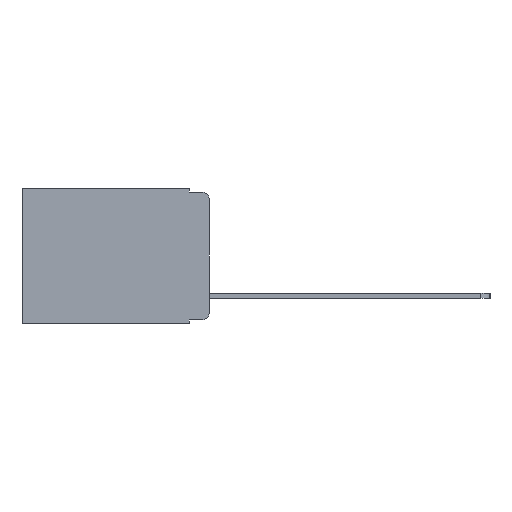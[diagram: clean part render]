
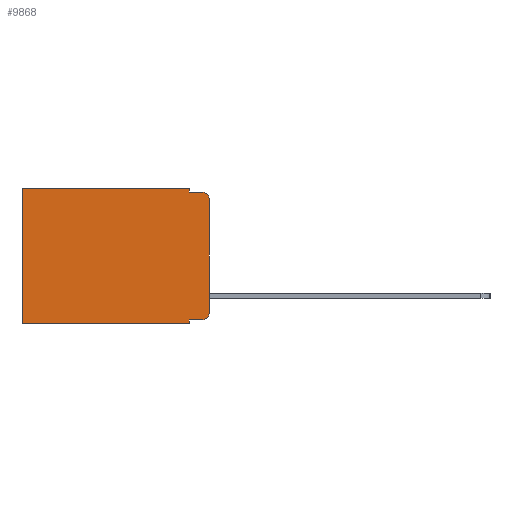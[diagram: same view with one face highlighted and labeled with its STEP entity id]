
A CAD part, left-side view. The second image highlights one B-rep face of the part: STEP entity #9868.
In plain terms, the highlighted planar face has unit normal (-1, 0, 0).
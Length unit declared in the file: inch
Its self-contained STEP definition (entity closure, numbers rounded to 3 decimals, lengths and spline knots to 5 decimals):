
#211 = CIRCLE ( 'NONE', #6795, 0.02 ) ;
#214 = DIRECTION ( 'NONE',  ( 0., 0., -1. ) ) ;
#392 = EDGE_LOOP ( 'NONE', ( #5761, #15468, #3379, #691, #3749, #3781, #10370, #563, #17552, #18116 ) ) ;
#563 = ORIENTED_EDGE ( 'NONE', *, *, #8234, .F. ) ;
#691 = ORIENTED_EDGE ( 'NONE', *, *, #2134, .F. ) ;
#769 = VERTEX_POINT ( 'NONE', #20588 ) ;
#883 = LINE ( 'NONE', #5434, #8383 ) ;
#1494 = CARTESIAN_POINT ( 'NONE',  ( 0.298, 0.051, -0.333 ) ) ;
#1606 = VERTEX_POINT ( 'NONE', #17451 ) ;
#1775 = CARTESIAN_POINT ( 'NONE',  ( 0.298, 0., -0.313 ) ) ;
#2134 = EDGE_CURVE ( 'NONE', #8348, #769, #4140, .T. ) ;
#2448 = LINE ( 'NONE', #13159, #6383 ) ;
#2516 = EDGE_CURVE ( 'NONE', #15425, #16596, #6400, .T. ) ;
#2732 = VECTOR ( 'NONE', #13446, 39.37008 ) ;
#3138 = CARTESIAN_POINT ( 'NONE',  ( 0.298, 0.051, 0. ) ) ;
#3336 = EDGE_CURVE ( 'NONE', #769, #10612, #2448, .T. ) ;
#3379 = ORIENTED_EDGE ( 'NONE', *, *, #3336, .F. ) ;
#3578 = CARTESIAN_POINT ( 'NONE',  ( 0.298, 0.051, -0.333 ) ) ;
#3749 = ORIENTED_EDGE ( 'NONE', *, *, #12738, .T. ) ;
#3781 = ORIENTED_EDGE ( 'NONE', *, *, #2516, .T. ) ;
#4140 = LINE ( 'NONE', #3138, #11976 ) ;
#4147 = CIRCLE ( 'NONE', #16805, 0.02 ) ;
#4214 = VERTEX_POINT ( 'NONE', #6397 ) ;
#4474 = VECTOR ( 'NONE', #13524, 39.37008 ) ;
#5371 = LINE ( 'NONE', #6850, #9315 ) ;
#5434 = CARTESIAN_POINT ( 'NONE',  ( 0.298, 0.051, 0. ) ) ;
#5755 = DIRECTION ( 'NONE',  ( 0., -1., 0. ) ) ;
#5761 = ORIENTED_EDGE ( 'NONE', *, *, #11861, .F. ) ;
#6383 = VECTOR ( 'NONE', #5755, 39.37008 ) ;
#6397 = CARTESIAN_POINT ( 'NONE',  ( 0.298, 0., -0.03 ) ) ;
#6400 = LINE ( 'NONE', #15675, #14639 ) ;
#6649 = FACE_OUTER_BOUND ( 'NONE', #392, .T. ) ;
#6795 = AXIS2_PLACEMENT_3D ( 'NONE', #17833, #8490, #19300 ) ;
#6850 = CARTESIAN_POINT ( 'NONE',  ( 0.298, 0., 0. ) ) ;
#6975 = DIRECTION ( 'NONE',  ( -1., 0., 0. ) ) ;
#7296 = CARTESIAN_POINT ( 'NONE',  ( 0.298, 0., 0. ) ) ;
#7990 = VERTEX_POINT ( 'NONE', #1494 ) ;
#8234 = EDGE_CURVE ( 'NONE', #7990, #1606, #883, .T. ) ;
#8348 = VERTEX_POINT ( 'NONE', #16875 ) ;
#8383 = VECTOR ( 'NONE', #214, 39.37008 ) ;
#8490 = DIRECTION ( 'NONE',  ( -1., 0., 0. ) ) ;
#8997 = DIRECTION ( 'NONE',  ( 1., 0., 0. ) ) ;
#9207 = CARTESIAN_POINT ( 'NONE',  ( 0.298, 0.02, -0.333 ) ) ;
#9315 = VECTOR ( 'NONE', #14993, 39.37008 ) ;
#9367 = VERTEX_POINT ( 'NONE', #9207 ) ;
#9449 = LINE ( 'NONE', #3578, #4474 ) ;
#9749 = EDGE_CURVE ( 'NONE', #9367, #16050, #211, .T. ) ;
#9868 = ADVANCED_FACE ( 'NONE', ( #6649 ), #16813, .F. ) ;
#10251 = VECTOR ( 'NONE', #19483, 39.37008 ) ;
#10370 = ORIENTED_EDGE ( 'NONE', *, *, #15253, .F. ) ;
#10612 = VERTEX_POINT ( 'NONE', #20762 ) ;
#11183 = CARTESIAN_POINT ( 'NONE',  ( 0.298, 0.473, -0.343 ) ) ;
#11581 = DIRECTION ( 'NONE',  ( 0., 0., -1. ) ) ;
#11861 = EDGE_CURVE ( 'NONE', #4214, #16050, #19175, .T. ) ;
#11976 = VECTOR ( 'NONE', #11581, 39.37008 ) ;
#12738 = EDGE_CURVE ( 'NONE', #8348, #15425, #5371, .T. ) ;
#13159 = CARTESIAN_POINT ( 'NONE',  ( 0.298, 0.051, -0.01 ) ) ;
#13446 = DIRECTION ( 'NONE',  ( 0., 0., -1. ) ) ;
#13524 = DIRECTION ( 'NONE',  ( 0., -1., 0. ) ) ;
#13968 = CARTESIAN_POINT ( 'NONE',  ( 0.298, 0.473, 0. ) ) ;
#14639 = VECTOR ( 'NONE', #17300, 39.37008 ) ;
#14993 = DIRECTION ( 'NONE',  ( 0., 1., 0. ) ) ;
#15253 = EDGE_CURVE ( 'NONE', #1606, #16596, #17922, .T. ) ;
#15425 = VERTEX_POINT ( 'NONE', #13968 ) ;
#15468 = ORIENTED_EDGE ( 'NONE', *, *, #19148, .T. ) ;
#15675 = CARTESIAN_POINT ( 'NONE',  ( 0.298, 0.473, 0. ) ) ;
#16044 = EDGE_CURVE ( 'NONE', #7990, #9367, #9449, .T. ) ;
#16050 = VERTEX_POINT ( 'NONE', #1775 ) ;
#16113 = AXIS2_PLACEMENT_3D ( 'NONE', #7296, #8997, #19743 ) ;
#16401 = CARTESIAN_POINT ( 'NONE',  ( 0.298, 0., 0. ) ) ;
#16551 = CARTESIAN_POINT ( 'NONE',  ( 0.298, 0.02, -0.03 ) ) ;
#16596 = VERTEX_POINT ( 'NONE', #11183 ) ;
#16805 = AXIS2_PLACEMENT_3D ( 'NONE', #16551, #6975, #18020 ) ;
#16813 = PLANE ( 'NONE',  #16113 ) ;
#16875 = CARTESIAN_POINT ( 'NONE',  ( 0.298, 0.051, 0. ) ) ;
#17300 = DIRECTION ( 'NONE',  ( 0., 0., -1. ) ) ;
#17451 = CARTESIAN_POINT ( 'NONE',  ( 0.298, 0.051, -0.343 ) ) ;
#17552 = ORIENTED_EDGE ( 'NONE', *, *, #16044, .T. ) ;
#17833 = CARTESIAN_POINT ( 'NONE',  ( 0.298, 0.02, -0.313 ) ) ;
#17922 = LINE ( 'NONE', #18028, #10251 ) ;
#18020 = DIRECTION ( 'NONE',  ( 0., 0., -1. ) ) ;
#18028 = CARTESIAN_POINT ( 'NONE',  ( 0.298, 0., -0.343 ) ) ;
#18116 = ORIENTED_EDGE ( 'NONE', *, *, #9749, .T. ) ;
#19148 = EDGE_CURVE ( 'NONE', #4214, #10612, #4147, .T. ) ;
#19175 = LINE ( 'NONE', #16401, #2732 ) ;
#19300 = DIRECTION ( 'NONE',  ( 0., 0., -1. ) ) ;
#19483 = DIRECTION ( 'NONE',  ( 0., 1., 0. ) ) ;
#19743 = DIRECTION ( 'NONE',  ( 0., 0., -1. ) ) ;
#20588 = CARTESIAN_POINT ( 'NONE',  ( 0.298, 0.051, -0.01 ) ) ;
#20762 = CARTESIAN_POINT ( 'NONE',  ( 0.298, 0.02, -0.01 ) ) ;
